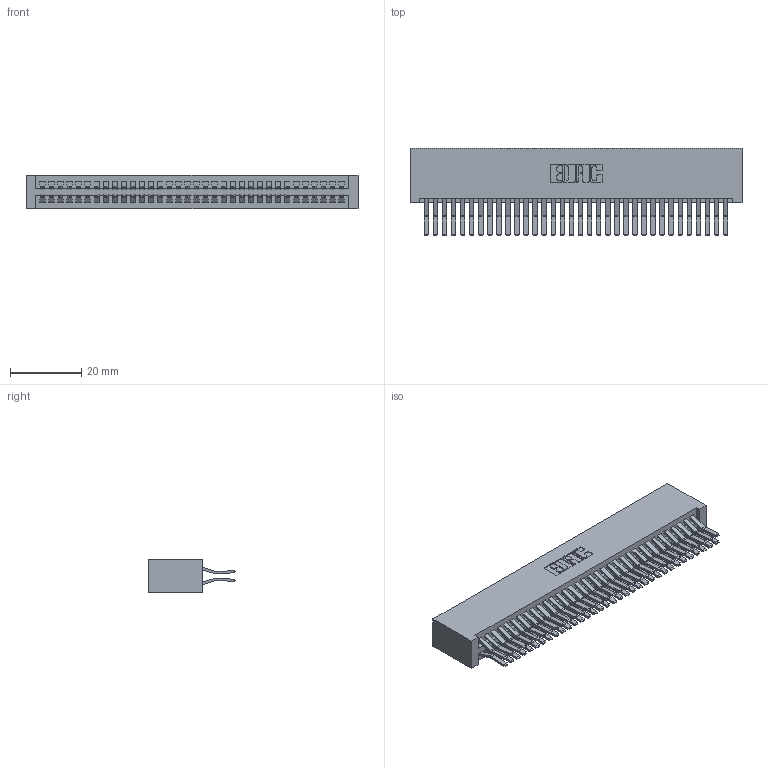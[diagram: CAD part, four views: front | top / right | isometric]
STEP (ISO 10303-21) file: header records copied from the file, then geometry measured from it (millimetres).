
FILE_DESCRIPTION (( 'STEP AP203' ), '1' );
FILE_NAME ('395-068-560-201.STEP', '2018-11-25T20:57:45', ( '' ), ( '' ), 'SwSTEP 2.0', 'SolidWorks 2016', '' );
FILE_SCHEMA (( 'CONFIG_CONTROL_DESIGN' ));
Length unit declared in the file: inch
Products named in the file (3): 395-068-560-201; 345 Part_No Mounting Lugs; 345-292-001_560 Tail
Assembly tree (69 placements, depth 2):
  395-068-560-201
    345 Part_No Mounting Lugs
    345-292-001_560 Tail  x68
Bounding box: 92.96 x 24.45 x 9.4 mm (x, y, z)
Volume: 10018 mm3; surface area: 16102.9 mm2
Topology: 69 solids, 69 shells, 3654 faces, 10857 edges, 7146 vertices
Faces by surface type: plane 2320, cylinder 1334
Entity records: 27565 total; most frequent: CARTESIAN_POINT 4628, ORIENTED_EDGE 4562, DIRECTION 4089, EDGE_CURVE 2281, VECTOR 2017, LINE 2017, VERTEX_POINT 1518, AXIS2_PLACEMENT_3D 1036
